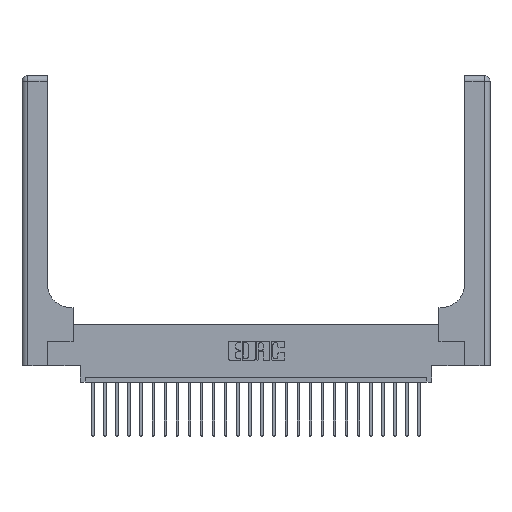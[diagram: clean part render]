
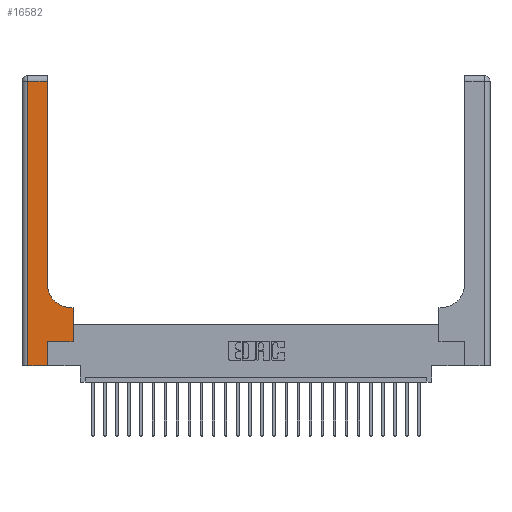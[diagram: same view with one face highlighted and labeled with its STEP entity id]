
A CAD part, top view. The second image highlights one B-rep face of the part: STEP entity #16582.
In plain terms, the highlighted planar face has unit normal (0, 0, 1).
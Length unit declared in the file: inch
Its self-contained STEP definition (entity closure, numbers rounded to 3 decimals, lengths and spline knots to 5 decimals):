
#110 = EDGE_LOOP ( 'NONE', ( #8751, #8040, #17914, #11327, #7179, #11287, #3408, #2374, #5755 ) ) ;
#115 = VECTOR ( 'NONE', #12364, 39.37008 ) ;
#291 = CARTESIAN_POINT ( 'NONE',  ( 0.265, 0., 0.37 ) ) ;
#789 = DIRECTION ( 'NONE',  ( 0., 1., 0. ) ) ;
#1614 = CARTESIAN_POINT ( 'NONE',  ( 0.06, 2.94, 0.37 ) ) ;
#2084 = VECTOR ( 'NONE', #12477, 39.37008 ) ;
#2374 = ORIENTED_EDGE ( 'NONE', *, *, #19582, .T. ) ;
#3324 = DIRECTION ( 'NONE',  ( -1., 0., 0. ) ) ;
#3405 = DIRECTION ( 'NONE',  ( 0., 0., -1. ) ) ;
#3408 = ORIENTED_EDGE ( 'NONE', *, *, #23353, .T. ) ;
#4248 = CARTESIAN_POINT ( 'NONE',  ( 0.265, 0.25, 0.37 ) ) ;
#4442 = EDGE_CURVE ( 'NONE', #7382, #11706, #12198, .T. ) ;
#5272 = CIRCLE ( 'NONE', #6917, 0.25 ) ;
#5684 = FACE_OUTER_BOUND ( 'NONE', #110, .T. ) ;
#5755 = ORIENTED_EDGE ( 'NONE', *, *, #24296, .T. ) ;
#6592 = CARTESIAN_POINT ( 'NONE',  ( 0.265, 0., 0.37 ) ) ;
#6917 = AXIS2_PLACEMENT_3D ( 'NONE', #22487, #24444, #11161 ) ;
#6973 = CARTESIAN_POINT ( 'NONE',  ( 0.528, 0.25, 0.37 ) ) ;
#7055 = CARTESIAN_POINT ( 'NONE',  ( 0., 3., 0.37 ) ) ;
#7152 = CARTESIAN_POINT ( 'NONE',  ( 0.26, 3., 0.37 ) ) ;
#7179 = ORIENTED_EDGE ( 'NONE', *, *, #13840, .T. ) ;
#7187 = VERTEX_POINT ( 'NONE', #16933 ) ;
#7382 = VERTEX_POINT ( 'NONE', #10011 ) ;
#7986 = LINE ( 'NONE', #7152, #2084 ) ;
#8040 = ORIENTED_EDGE ( 'NONE', *, *, #4442, .T. ) ;
#8557 = VECTOR ( 'NONE', #22492, 39.37008 ) ;
#8751 = ORIENTED_EDGE ( 'NONE', *, *, #22033, .T. ) ;
#8801 = CARTESIAN_POINT ( 'NONE',  ( 0., 2.94, 0.37 ) ) ;
#10011 = CARTESIAN_POINT ( 'NONE',  ( 0.26, 2.94, 0.37 ) ) ;
#10289 = LINE ( 'NONE', #291, #12672 ) ;
#10479 = VERTEX_POINT ( 'NONE', #13877 ) ;
#10659 = LINE ( 'NONE', #23099, #22198 ) ;
#11161 = DIRECTION ( 'NONE',  ( 1., 0., 0. ) ) ;
#11287 = ORIENTED_EDGE ( 'NONE', *, *, #11606, .T. ) ;
#11327 = ORIENTED_EDGE ( 'NONE', *, *, #12483, .T. ) ;
#11332 = CARTESIAN_POINT ( 'NONE',  ( 0.528, 0.6, 0.37 ) ) ;
#11606 = EDGE_CURVE ( 'NONE', #24020, #17972, #12139, .T. ) ;
#11706 = VERTEX_POINT ( 'NONE', #1614 ) ;
#11932 = DIRECTION ( 'NONE',  ( 0., -1., 0. ) ) ;
#11990 = EDGE_CURVE ( 'NONE', #11706, #7187, #14183, .T. ) ;
#12139 = LINE ( 'NONE', #17970, #24010 ) ;
#12198 = LINE ( 'NONE', #8801, #16340 ) ;
#12364 = DIRECTION ( 'NONE',  ( -1., 0., 0. ) ) ;
#12477 = DIRECTION ( 'NONE',  ( 0., 1., 0. ) ) ;
#12483 = EDGE_CURVE ( 'NONE', #7187, #15144, #10659, .T. ) ;
#12672 = VECTOR ( 'NONE', #789, 39.37008 ) ;
#12806 = VERTEX_POINT ( 'NONE', #11332 ) ;
#13580 = DIRECTION ( 'NONE',  ( 1., 0., 0. ) ) ;
#13665 = CARTESIAN_POINT ( 'NONE',  ( 0.06, 3., 0.37 ) ) ;
#13840 = EDGE_CURVE ( 'NONE', #15144, #24020, #10289, .T. ) ;
#13877 = CARTESIAN_POINT ( 'NONE',  ( 0.51, 0.6, 0.37 ) ) ;
#14183 = LINE ( 'NONE', #13665, #16596 ) ;
#14737 = PLANE ( 'NONE',  #22042 ) ;
#14764 = LINE ( 'NONE', #18372, #8557 ) ;
#15144 = VERTEX_POINT ( 'NONE', #6592 ) ;
#16340 = VECTOR ( 'NONE', #19827, 39.37008 ) ;
#16582 = ADVANCED_FACE ( 'NONE', ( #5684 ), #14737, .F. ) ;
#16596 = VECTOR ( 'NONE', #11932, 39.37008 ) ;
#16933 = CARTESIAN_POINT ( 'NONE',  ( 0.06, 0., 0.37 ) ) ;
#17914 = ORIENTED_EDGE ( 'NONE', *, *, #11990, .T. ) ;
#17970 = CARTESIAN_POINT ( 'NONE',  ( 0.265, 0.25, 0.37 ) ) ;
#17972 = VERTEX_POINT ( 'NONE', #6973 ) ;
#17999 = VERTEX_POINT ( 'NONE', #20881 ) ;
#18372 = CARTESIAN_POINT ( 'NONE',  ( 0.528, 0.25, 0.37 ) ) ;
#19582 = EDGE_CURVE ( 'NONE', #12806, #10479, #22942, .T. ) ;
#19827 = DIRECTION ( 'NONE',  ( -1., 0., 0. ) ) ;
#20124 = CARTESIAN_POINT ( 'NONE',  ( 0.26, 0.6, 0.37 ) ) ;
#20881 = CARTESIAN_POINT ( 'NONE',  ( 0.26, 0.85, 0.37 ) ) ;
#22033 = EDGE_CURVE ( 'NONE', #17999, #7382, #7986, .T. ) ;
#22042 = AXIS2_PLACEMENT_3D ( 'NONE', #7055, #3405, #3324 ) ;
#22198 = VECTOR ( 'NONE', #13580, 39.37008 ) ;
#22487 = CARTESIAN_POINT ( 'NONE',  ( 0.51, 0.85, 0.37 ) ) ;
#22492 = DIRECTION ( 'NONE',  ( 0., 1., 0. ) ) ;
#22942 = LINE ( 'NONE', #20124, #115 ) ;
#23099 = CARTESIAN_POINT ( 'NONE',  ( 0., 0., 0.37 ) ) ;
#23353 = EDGE_CURVE ( 'NONE', #17972, #12806, #14764, .T. ) ;
#23952 = DIRECTION ( 'NONE',  ( 1., 0., 0. ) ) ;
#24010 = VECTOR ( 'NONE', #23952, 39.37008 ) ;
#24020 = VERTEX_POINT ( 'NONE', #4248 ) ;
#24296 = EDGE_CURVE ( 'NONE', #10479, #17999, #5272, .T. ) ;
#24444 = DIRECTION ( 'NONE',  ( 0., 0., -1. ) ) ;
